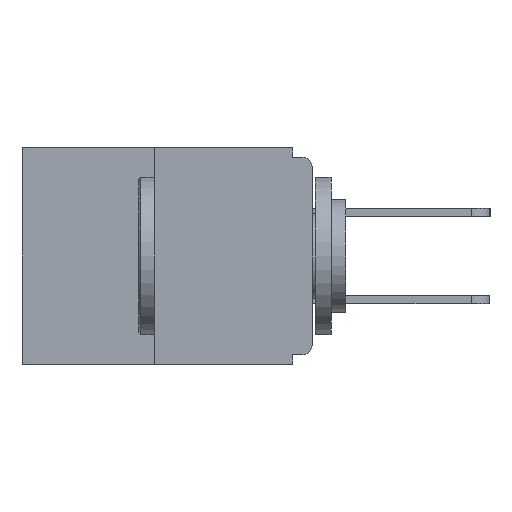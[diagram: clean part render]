
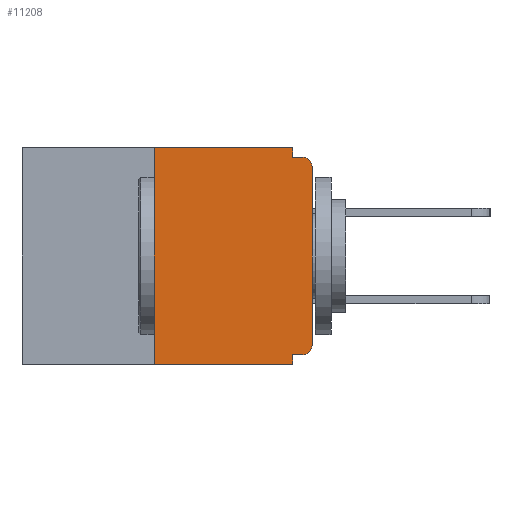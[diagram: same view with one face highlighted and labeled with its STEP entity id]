
A CAD part, left-side view. The second image highlights one B-rep face of the part: STEP entity #11208.
In plain terms, the highlighted planar face has unit normal (-1, 0, 0).
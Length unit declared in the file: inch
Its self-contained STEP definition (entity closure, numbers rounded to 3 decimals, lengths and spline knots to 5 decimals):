
#628 = EDGE_CURVE ( 'NONE', #2576, #1838, #12718, .T. ) ;
#655 = PLANE ( 'NONE',  #7687 ) ;
#721 = ORIENTED_EDGE ( 'NONE', *, *, #11310, .F. ) ;
#1021 = DIRECTION ( 'NONE',  ( 0., -1., 0. ) ) ;
#1087 = VECTOR ( 'NONE', #15142, 39.37008 ) ;
#1838 = VERTEX_POINT ( 'NONE', #20751 ) ;
#2245 = VERTEX_POINT ( 'NONE', #27748 ) ;
#2576 = VERTEX_POINT ( 'NONE', #4515 ) ;
#2912 = VERTEX_POINT ( 'NONE', #14661 ) ;
#2916 = CARTESIAN_POINT ( 'NONE',  ( 0., 0.46, 0. ) ) ;
#3376 = VERTEX_POINT ( 'NONE', #25478 ) ;
#3484 = VECTOR ( 'NONE', #7389, 39.37008 ) ;
#4235 = AXIS2_PLACEMENT_3D ( 'NONE', #29117, #18184, #18095 ) ;
#4515 = CARTESIAN_POINT ( 'NONE',  ( 0., 0., -0.313 ) ) ;
#5732 = ORIENTED_EDGE ( 'NONE', *, *, #20389, .T. ) ;
#5970 = VECTOR ( 'NONE', #1021, 39.37008 ) ;
#6058 = ORIENTED_EDGE ( 'NONE', *, *, #23247, .F. ) ;
#6101 = DIRECTION ( 'NONE',  ( 0., 0., -1. ) ) ;
#6260 = CARTESIAN_POINT ( 'NONE',  ( 0., 0.031, -0.328 ) ) ;
#7322 = DIRECTION ( 'NONE',  ( -1., 0., 0. ) ) ;
#7389 = DIRECTION ( 'NONE',  ( 0., -1., 0. ) ) ;
#7422 = CARTESIAN_POINT ( 'NONE',  ( 0., 0.015, -0.313 ) ) ;
#7687 = AXIS2_PLACEMENT_3D ( 'NONE', #18872, #9779, #12067 ) ;
#8545 = LINE ( 'NONE', #17942, #13829 ) ;
#8769 = EDGE_CURVE ( 'NONE', #1838, #29090, #29153, .T. ) ;
#8844 = VECTOR ( 'NONE', #13533, 39.37008 ) ;
#8932 = DIRECTION ( 'NONE',  ( 0., 1., 0. ) ) ;
#9304 = DIRECTION ( 'NONE',  ( 0., 0., -1. ) ) ;
#9779 = DIRECTION ( 'NONE',  ( 1., 0., 0. ) ) ;
#10199 = CIRCLE ( 'NONE', #16270, 0.015 ) ;
#10339 = LINE ( 'NONE', #12871, #1087 ) ;
#10490 = CARTESIAN_POINT ( 'NONE',  ( 0., 0.25, 0. ) ) ;
#10772 = CARTESIAN_POINT ( 'NONE',  ( 0., 0.031, -0.343 ) ) ;
#10957 = LINE ( 'NONE', #10490, #15919 ) ;
#11192 = ORIENTED_EDGE ( 'NONE', *, *, #14852, .F. ) ;
#11208 = ADVANCED_FACE ( 'NONE', ( #19103 ), #655, .F. ) ;
#11272 = CARTESIAN_POINT ( 'NONE',  ( 0., 0., 0. ) ) ;
#11310 = EDGE_CURVE ( 'NONE', #17874, #16838, #21545, .T. ) ;
#12067 = DIRECTION ( 'NONE',  ( 0., 0., -1. ) ) ;
#12718 = LINE ( 'NONE', #11272, #8844 ) ;
#12871 = CARTESIAN_POINT ( 'NONE',  ( 0., 0.031, 0. ) ) ;
#13533 = DIRECTION ( 'NONE',  ( 0., 0., 1. ) ) ;
#13829 = VECTOR ( 'NONE', #26717, 39.37008 ) ;
#13876 = ORIENTED_EDGE ( 'NONE', *, *, #28286, .F. ) ;
#14349 = VERTEX_POINT ( 'NONE', #24742 ) ;
#14661 = CARTESIAN_POINT ( 'NONE',  ( 0., 0.031, 0. ) ) ;
#14852 = EDGE_CURVE ( 'NONE', #2912, #3376, #10339, .T. ) ;
#15142 = DIRECTION ( 'NONE',  ( 0., 0., -1. ) ) ;
#15624 = ORIENTED_EDGE ( 'NONE', *, *, #28703, .F. ) ;
#15919 = VECTOR ( 'NONE', #26265, 39.37008 ) ;
#16270 = AXIS2_PLACEMENT_3D ( 'NONE', #7422, #7322, #9304 ) ;
#16776 = CARTESIAN_POINT ( 'NONE',  ( 0., 0., -0.015 ) ) ;
#16838 = VERTEX_POINT ( 'NONE', #20211 ) ;
#17295 = CARTESIAN_POINT ( 'NONE',  ( 0., 0.015, -0.015 ) ) ;
#17874 = VERTEX_POINT ( 'NONE', #6260 ) ;
#17942 = CARTESIAN_POINT ( 'NONE',  ( 0., 0.46, -0.343 ) ) ;
#18095 = DIRECTION ( 'NONE',  ( 0., 0., -1. ) ) ;
#18184 = DIRECTION ( 'NONE',  ( -1., 0., 0. ) ) ;
#18872 = CARTESIAN_POINT ( 'NONE',  ( 0., 0.46, 0. ) ) ;
#19039 = LINE ( 'NONE', #2916, #3484 ) ;
#19103 = FACE_OUTER_BOUND ( 'NONE', #25496, .T. ) ;
#19387 = ORIENTED_EDGE ( 'NONE', *, *, #628, .T. ) ;
#20211 = CARTESIAN_POINT ( 'NONE',  ( 0., 0.031, -0.343 ) ) ;
#20389 = EDGE_CURVE ( 'NONE', #25911, #2576, #10199, .T. ) ;
#20454 = CARTESIAN_POINT ( 'NONE',  ( 0., 0.015, -0.328 ) ) ;
#20751 = CARTESIAN_POINT ( 'NONE',  ( 0., 0., -0.03 ) ) ;
#21277 = LINE ( 'NONE', #26795, #28680 ) ;
#21381 = ORIENTED_EDGE ( 'NONE', *, *, #27863, .F. ) ;
#21545 = LINE ( 'NONE', #10772, #27571 ) ;
#22490 = ORIENTED_EDGE ( 'NONE', *, *, #8769, .T. ) ;
#23247 = EDGE_CURVE ( 'NONE', #2245, #2912, #19039, .T. ) ;
#24742 = CARTESIAN_POINT ( 'NONE',  ( 0., 0.25, -0.343 ) ) ;
#25456 = LINE ( 'NONE', #16776, #5970 ) ;
#25478 = CARTESIAN_POINT ( 'NONE',  ( 0., 0.031, -0.015 ) ) ;
#25496 = EDGE_LOOP ( 'NONE', ( #6058, #13876, #29140, #721, #21381, #5732, #19387, #22490, #15624, #11192 ) ) ;
#25911 = VERTEX_POINT ( 'NONE', #20454 ) ;
#26265 = DIRECTION ( 'NONE',  ( 0., 0., 1. ) ) ;
#26717 = DIRECTION ( 'NONE',  ( 0., -1., 0. ) ) ;
#26795 = CARTESIAN_POINT ( 'NONE',  ( 0., 0., -0.328 ) ) ;
#27338 = EDGE_CURVE ( 'NONE', #14349, #16838, #8545, .T. ) ;
#27571 = VECTOR ( 'NONE', #6101, 39.37008 ) ;
#27748 = CARTESIAN_POINT ( 'NONE',  ( 0., 0.25, 0. ) ) ;
#27863 = EDGE_CURVE ( 'NONE', #25911, #17874, #21277, .T. ) ;
#28286 = EDGE_CURVE ( 'NONE', #14349, #2245, #10957, .T. ) ;
#28680 = VECTOR ( 'NONE', #8932, 39.37008 ) ;
#28703 = EDGE_CURVE ( 'NONE', #3376, #29090, #25456, .T. ) ;
#29090 = VERTEX_POINT ( 'NONE', #17295 ) ;
#29117 = CARTESIAN_POINT ( 'NONE',  ( 0., 0.015, -0.03 ) ) ;
#29140 = ORIENTED_EDGE ( 'NONE', *, *, #27338, .T. ) ;
#29153 = CIRCLE ( 'NONE', #4235, 0.015 ) ;
